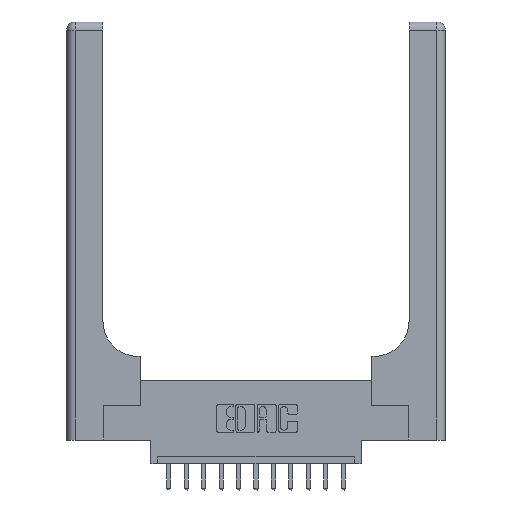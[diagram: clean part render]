
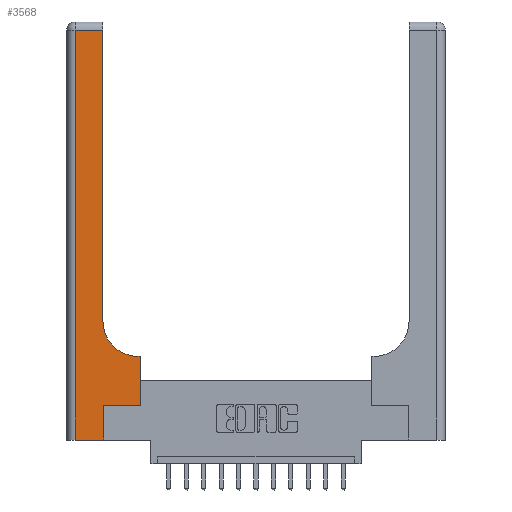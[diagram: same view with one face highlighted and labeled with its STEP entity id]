
A CAD part, top view. The second image highlights one B-rep face of the part: STEP entity #3568.
In plain terms, the highlighted planar face has unit normal (0, 0, 1).
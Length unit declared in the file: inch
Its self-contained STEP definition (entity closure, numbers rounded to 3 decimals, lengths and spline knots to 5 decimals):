
#92 = PLANE ( 'NONE',  #4753 ) ;
#118 = CARTESIAN_POINT ( 'NONE',  ( 0.26, 0.85, 0.37 ) ) ;
#331 = VERTEX_POINT ( 'NONE', #11026 ) ;
#379 = EDGE_CURVE ( 'NONE', #331, #8676, #3279, .T. ) ;
#461 = ORIENTED_EDGE ( 'NONE', *, *, #4354, .T. ) ;
#693 = VECTOR ( 'NONE', #11868, 39.37008 ) ;
#694 = CIRCLE ( 'NONE', #13765, 0.25 ) ;
#713 = EDGE_CURVE ( 'NONE', #14200, #6999, #6230, .T. ) ;
#1271 = FACE_OUTER_BOUND ( 'NONE', #13541, .T. ) ;
#1436 = CARTESIAN_POINT ( 'NONE',  ( 0., 3., 0.37 ) ) ;
#1716 = CARTESIAN_POINT ( 'NONE',  ( 0.265, 0., 0.37 ) ) ;
#1993 = LINE ( 'NONE', #4381, #14254 ) ;
#2170 = LINE ( 'NONE', #16675, #15622 ) ;
#2721 = EDGE_CURVE ( 'NONE', #10461, #11313, #10066, .T. ) ;
#3178 = LINE ( 'NONE', #1716, #4774 ) ;
#3279 = LINE ( 'NONE', #13671, #8200 ) ;
#3443 = DIRECTION ( 'NONE',  ( -1., 0., 0. ) ) ;
#3568 = ADVANCED_FACE ( 'NONE', ( #1271 ), #92, .F. ) ;
#3671 = DIRECTION ( 'NONE',  ( 0., 0., -1. ) ) ;
#3775 = VERTEX_POINT ( 'NONE', #14820 ) ;
#3833 = DIRECTION ( 'NONE',  ( 1., 0., 0. ) ) ;
#3993 = CARTESIAN_POINT ( 'NONE',  ( 0.528, 0.25, 0.37 ) ) ;
#4354 = EDGE_CURVE ( 'NONE', #5454, #331, #2170, .T. ) ;
#4381 = CARTESIAN_POINT ( 'NONE',  ( 0.06, 3., 0.37 ) ) ;
#4753 = AXIS2_PLACEMENT_3D ( 'NONE', #1436, #3671, #16877 ) ;
#4774 = VECTOR ( 'NONE', #8215, 39.37008 ) ;
#4927 = DIRECTION ( 'NONE',  ( 1., 0., 0. ) ) ;
#5153 = ORIENTED_EDGE ( 'NONE', *, *, #379, .T. ) ;
#5454 = VERTEX_POINT ( 'NONE', #118 ) ;
#6145 = CARTESIAN_POINT ( 'NONE',  ( 0.51, 0.85, 0.37 ) ) ;
#6230 = LINE ( 'NONE', #15507, #13360 ) ;
#6561 = CARTESIAN_POINT ( 'NONE',  ( 0.265, 0.25, 0.37 ) ) ;
#6923 = CARTESIAN_POINT ( 'NONE',  ( 0.265, 0., 0.37 ) ) ;
#6999 = VERTEX_POINT ( 'NONE', #6923 ) ;
#7234 = ORIENTED_EDGE ( 'NONE', *, *, #15211, .T. ) ;
#7339 = ORIENTED_EDGE ( 'NONE', *, *, #2721, .T. ) ;
#7392 = ORIENTED_EDGE ( 'NONE', *, *, #13202, .T. ) ;
#7524 = DIRECTION ( 'NONE',  ( 1., 0., 0. ) ) ;
#7638 = ORIENTED_EDGE ( 'NONE', *, *, #713, .T. ) ;
#7988 = LINE ( 'NONE', #15542, #693 ) ;
#8054 = ORIENTED_EDGE ( 'NONE', *, *, #16491, .T. ) ;
#8200 = VECTOR ( 'NONE', #3443, 39.37008 ) ;
#8215 = DIRECTION ( 'NONE',  ( 0., 1., 0. ) ) ;
#8347 = VERTEX_POINT ( 'NONE', #12702 ) ;
#8676 = VERTEX_POINT ( 'NONE', #13957 ) ;
#8881 = CARTESIAN_POINT ( 'NONE',  ( 0.265, 0.25, 0.37 ) ) ;
#8926 = DIRECTION ( 'NONE',  ( 0., 1., 0. ) ) ;
#8963 = VECTOR ( 'NONE', #4927, 39.37008 ) ;
#9692 = DIRECTION ( 'NONE',  ( 0., -1., 0. ) ) ;
#10066 = LINE ( 'NONE', #8881, #8963 ) ;
#10388 = DIRECTION ( 'NONE',  ( 0., 1., 0. ) ) ;
#10461 = VERTEX_POINT ( 'NONE', #6561 ) ;
#10527 = EDGE_CURVE ( 'NONE', #11313, #3775, #15665, .T. ) ;
#11026 = CARTESIAN_POINT ( 'NONE',  ( 0.26, 2.94, 0.37 ) ) ;
#11313 = VERTEX_POINT ( 'NONE', #14107 ) ;
#11373 = CARTESIAN_POINT ( 'NONE',  ( 0.06, 0., 0.37 ) ) ;
#11868 = DIRECTION ( 'NONE',  ( -1., 0., 0. ) ) ;
#12702 = CARTESIAN_POINT ( 'NONE',  ( 0.51, 0.6, 0.37 ) ) ;
#12991 = ORIENTED_EDGE ( 'NONE', *, *, #10527, .T. ) ;
#13202 = EDGE_CURVE ( 'NONE', #8347, #5454, #694, .T. ) ;
#13360 = VECTOR ( 'NONE', #3833, 39.37008 ) ;
#13407 = VECTOR ( 'NONE', #10388, 39.37008 ) ;
#13541 = EDGE_LOOP ( 'NONE', ( #461, #5153, #8054, #7638, #13700, #7339, #12991, #7234, #7392 ) ) ;
#13671 = CARTESIAN_POINT ( 'NONE',  ( 0., 2.94, 0.37 ) ) ;
#13700 = ORIENTED_EDGE ( 'NONE', *, *, #15681, .T. ) ;
#13765 = AXIS2_PLACEMENT_3D ( 'NONE', #6145, #13991, #7524 ) ;
#13957 = CARTESIAN_POINT ( 'NONE',  ( 0.06, 2.94, 0.37 ) ) ;
#13991 = DIRECTION ( 'NONE',  ( 0., 0., -1. ) ) ;
#14107 = CARTESIAN_POINT ( 'NONE',  ( 0.528, 0.25, 0.37 ) ) ;
#14200 = VERTEX_POINT ( 'NONE', #11373 ) ;
#14254 = VECTOR ( 'NONE', #9692, 39.37008 ) ;
#14820 = CARTESIAN_POINT ( 'NONE',  ( 0.528, 0.6, 0.37 ) ) ;
#15211 = EDGE_CURVE ( 'NONE', #3775, #8347, #7988, .T. ) ;
#15507 = CARTESIAN_POINT ( 'NONE',  ( 0., 0., 0.37 ) ) ;
#15542 = CARTESIAN_POINT ( 'NONE',  ( 0.26, 0.6, 0.37 ) ) ;
#15622 = VECTOR ( 'NONE', #8926, 39.37008 ) ;
#15665 = LINE ( 'NONE', #3993, #13407 ) ;
#15681 = EDGE_CURVE ( 'NONE', #6999, #10461, #3178, .T. ) ;
#16491 = EDGE_CURVE ( 'NONE', #8676, #14200, #1993, .T. ) ;
#16675 = CARTESIAN_POINT ( 'NONE',  ( 0.26, 3., 0.37 ) ) ;
#16877 = DIRECTION ( 'NONE',  ( -1., 0., 0. ) ) ;
